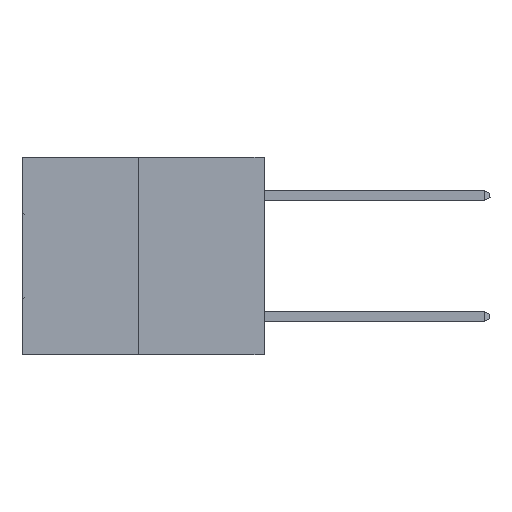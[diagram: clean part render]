
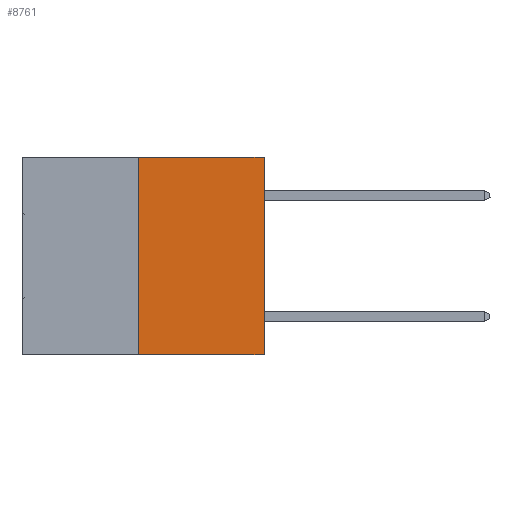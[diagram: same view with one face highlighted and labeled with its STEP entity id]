
A CAD part, left-side view. The second image highlights one B-rep face of the part: STEP entity #8761.
In plain terms, the highlighted planar face has unit normal (-1, 0, 0).
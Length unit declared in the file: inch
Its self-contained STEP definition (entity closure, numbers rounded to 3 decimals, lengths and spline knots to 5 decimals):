
#1873 = AXIS2_PLACEMENT_3D ( 'NONE', #31686, #25959, #5524 ) ;
#2599 = CARTESIAN_POINT ( 'NONE',  ( 0., 0.6, -0.49 ) ) ;
#4245 = VERTEX_POINT ( 'NONE', #34031 ) ;
#4698 = EDGE_LOOP ( 'NONE', ( #23505, #17920, #5572, #5239 ) ) ;
#5239 = ORIENTED_EDGE ( 'NONE', *, *, #16718, .F. ) ;
#5524 = DIRECTION ( 'NONE',  ( 0., 0., -1. ) ) ;
#5572 = ORIENTED_EDGE ( 'NONE', *, *, #27102, .T. ) ;
#8426 = LINE ( 'NONE', #15592, #9337 ) ;
#8761 = ADVANCED_FACE ( 'NONE', ( #29019 ), #34354, .F. ) ;
#9337 = VECTOR ( 'NONE', #12849, 39.37008 ) ;
#9842 = CARTESIAN_POINT ( 'NONE',  ( 0., 0., 0. ) ) ;
#10619 = LINE ( 'NONE', #2599, #14695 ) ;
#12849 = DIRECTION ( 'NONE',  ( 0., 0., 1. ) ) ;
#14695 = VECTOR ( 'NONE', #19825, 39.37008 ) ;
#15592 = CARTESIAN_POINT ( 'NONE',  ( 0., 0.312, -0.49 ) ) ;
#16718 = EDGE_CURVE ( 'NONE', #26701, #18946, #22504, .T. ) ;
#17022 = EDGE_CURVE ( 'NONE', #4245, #26701, #8426, .T. ) ;
#17920 = ORIENTED_EDGE ( 'NONE', *, *, #22065, .T. ) ;
#18946 = VERTEX_POINT ( 'NONE', #9842 ) ;
#19300 = VECTOR ( 'NONE', #29157, 39.37008 ) ;
#19825 = DIRECTION ( 'NONE',  ( 0., -1., 0. ) ) ;
#22065 = EDGE_CURVE ( 'NONE', #4245, #33187, #10619, .T. ) ;
#22504 = LINE ( 'NONE', #31314, #29277 ) ;
#23181 = CARTESIAN_POINT ( 'NONE',  ( 0., 0.312, 0. ) ) ;
#23505 = ORIENTED_EDGE ( 'NONE', *, *, #17022, .F. ) ;
#25959 = DIRECTION ( 'NONE',  ( 1., 0., 0. ) ) ;
#26701 = VERTEX_POINT ( 'NONE', #23181 ) ;
#27102 = EDGE_CURVE ( 'NONE', #33187, #18946, #34251, .T. ) ;
#29019 = FACE_OUTER_BOUND ( 'NONE', #4698, .T. ) ;
#29157 = DIRECTION ( 'NONE',  ( 0., 0., 1. ) ) ;
#29277 = VECTOR ( 'NONE', #34347, 39.37008 ) ;
#29300 = CARTESIAN_POINT ( 'NONE',  ( 0., 0., 0. ) ) ;
#31314 = CARTESIAN_POINT ( 'NONE',  ( 0., 0.6, 0. ) ) ;
#31686 = CARTESIAN_POINT ( 'NONE',  ( 0., 0.6, 0. ) ) ;
#33187 = VERTEX_POINT ( 'NONE', #35596 ) ;
#34031 = CARTESIAN_POINT ( 'NONE',  ( 0., 0.312, -0.49 ) ) ;
#34251 = LINE ( 'NONE', #29300, #19300 ) ;
#34347 = DIRECTION ( 'NONE',  ( 0., -1., 0. ) ) ;
#34354 = PLANE ( 'NONE',  #1873 ) ;
#35596 = CARTESIAN_POINT ( 'NONE',  ( 0., 0., -0.49 ) ) ;
